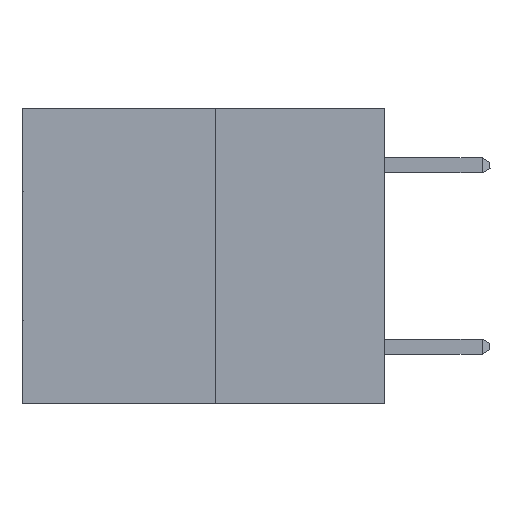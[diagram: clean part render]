
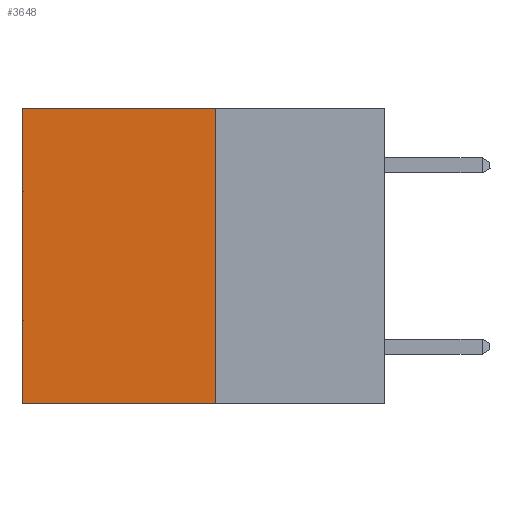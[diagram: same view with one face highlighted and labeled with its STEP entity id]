
A CAD part, left-side view. The second image highlights one B-rep face of the part: STEP entity #3648.
In plain terms, the highlighted planar face has unit normal (-1, 0, 0).
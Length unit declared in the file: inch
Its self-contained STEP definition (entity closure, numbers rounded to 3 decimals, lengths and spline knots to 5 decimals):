
#606 = VERTEX_POINT ( 'NONE', #9154 ) ;
#1857 = LINE ( 'NONE', #6544, #27529 ) ;
#1914 = VERTEX_POINT ( 'NONE', #27126 ) ;
#3648 = ADVANCED_FACE ( 'NONE', ( #19866 ), #24301, .F. ) ;
#4659 = AXIS2_PLACEMENT_3D ( 'NONE', #26722, #29192, #9679 ) ;
#6544 = CARTESIAN_POINT ( 'NONE',  ( 0.3165, 0.6, -0.49 ) ) ;
#6804 = VERTEX_POINT ( 'NONE', #25763 ) ;
#7998 = EDGE_CURVE ( 'NONE', #6804, #1914, #30683, .T. ) ;
#8222 = EDGE_CURVE ( 'NONE', #19552, #606, #28750, .T. ) ;
#8783 = CARTESIAN_POINT ( 'NONE',  ( 0.3165, 0.28, -0.49 ) ) ;
#9154 = CARTESIAN_POINT ( 'NONE',  ( 0.3165, 0.6, 0. ) ) ;
#9679 = DIRECTION ( 'NONE',  ( 0., 0., -1. ) ) ;
#9901 = DIRECTION ( 'NONE',  ( 0., 1., 0. ) ) ;
#14278 = EDGE_LOOP ( 'NONE', ( #17024, #26298, #28954, #23273 ) ) ;
#15567 = CARTESIAN_POINT ( 'NONE',  ( 0.3165, 0.28, 0. ) ) ;
#16080 = CARTESIAN_POINT ( 'NONE',  ( 0.3165, 0.28, -0.49 ) ) ;
#17024 = ORIENTED_EDGE ( 'NONE', *, *, #30380, .T. ) ;
#19552 = VERTEX_POINT ( 'NONE', #15567 ) ;
#19866 = FACE_OUTER_BOUND ( 'NONE', #14278, .T. ) ;
#21567 = VECTOR ( 'NONE', #9901, 39.37008 ) ;
#21604 = VECTOR ( 'NONE', #23731, 39.37008 ) ;
#23273 = ORIENTED_EDGE ( 'NONE', *, *, #8222, .T. ) ;
#23444 = VECTOR ( 'NONE', #30320, 39.37008 ) ;
#23513 = DIRECTION ( 'NONE',  ( 0., 0., -1. ) ) ;
#23731 = DIRECTION ( 'NONE',  ( 0., 0., -1. ) ) ;
#24301 = PLANE ( 'NONE',  #4659 ) ;
#24644 = CARTESIAN_POINT ( 'NONE',  ( 0.3165, 0.28, 0. ) ) ;
#25763 = CARTESIAN_POINT ( 'NONE',  ( 0.3165, 0.28, -0.49 ) ) ;
#26298 = ORIENTED_EDGE ( 'NONE', *, *, #7998, .F. ) ;
#26722 = CARTESIAN_POINT ( 'NONE',  ( 0.3165, 0.28, -0.49 ) ) ;
#27126 = CARTESIAN_POINT ( 'NONE',  ( 0.3165, 0.6, -0.49 ) ) ;
#27529 = VECTOR ( 'NONE', #23513, 39.37008 ) ;
#28750 = LINE ( 'NONE', #24644, #21567 ) ;
#28753 = EDGE_CURVE ( 'NONE', #19552, #6804, #31115, .T. ) ;
#28954 = ORIENTED_EDGE ( 'NONE', *, *, #28753, .F. ) ;
#29192 = DIRECTION ( 'NONE',  ( 1., 0., 0. ) ) ;
#30320 = DIRECTION ( 'NONE',  ( 0., 1., 0. ) ) ;
#30380 = EDGE_CURVE ( 'NONE', #606, #1914, #1857, .T. ) ;
#30683 = LINE ( 'NONE', #8783, #23444 ) ;
#31115 = LINE ( 'NONE', #16080, #21604 ) ;
